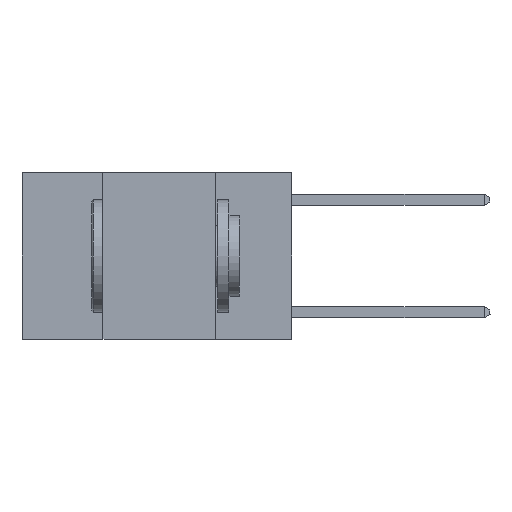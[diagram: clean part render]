
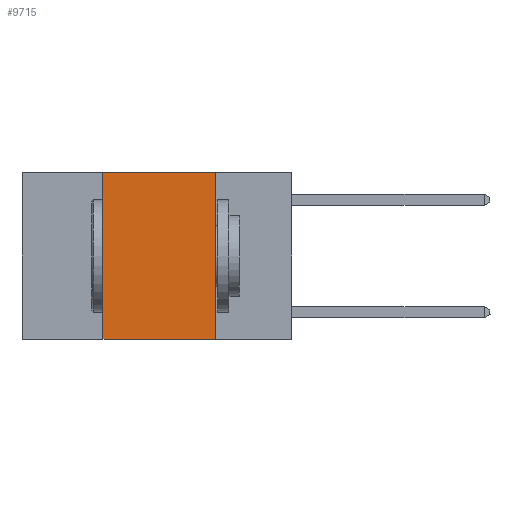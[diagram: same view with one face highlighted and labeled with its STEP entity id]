
A CAD part, left-side view. The second image highlights one B-rep face of the part: STEP entity #9715.
In plain terms, the highlighted planar face has unit normal (-1, 0, 0).
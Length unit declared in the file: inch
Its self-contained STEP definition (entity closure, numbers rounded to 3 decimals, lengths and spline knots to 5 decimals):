
#93 = DIRECTION ( 'NONE',  ( 1., 0., 0. ) ) ;
#131 = LINE ( 'NONE', #6409, #14704 ) ;
#371 = EDGE_LOOP ( 'NONE', ( #15436, #6193, #489, #10617 ) ) ;
#489 = ORIENTED_EDGE ( 'NONE', *, *, #5505, .F. ) ;
#572 = AXIS2_PLACEMENT_3D ( 'NONE', #1726, #93, #17816 ) ;
#579 = LINE ( 'NONE', #14500, #13747 ) ;
#1726 = CARTESIAN_POINT ( 'NONE',  ( 0., 0.6, 0. ) ) ;
#3951 = VERTEX_POINT ( 'NONE', #20063 ) ;
#4758 = CARTESIAN_POINT ( 'NONE',  ( 0., 0.6, -0.37 ) ) ;
#5505 = EDGE_CURVE ( 'NONE', #15310, #16180, #8501, .T. ) ;
#5695 = VERTEX_POINT ( 'NONE', #18073 ) ;
#6193 = ORIENTED_EDGE ( 'NONE', *, *, #14468, .F. ) ;
#6409 = CARTESIAN_POINT ( 'NONE',  ( 0., 0.17, 0. ) ) ;
#6821 = DIRECTION ( 'NONE',  ( 0., 0., 1. ) ) ;
#7764 = DIRECTION ( 'NONE',  ( 0., -1., 0. ) ) ;
#8501 = LINE ( 'NONE', #9853, #15175 ) ;
#8723 = EDGE_CURVE ( 'NONE', #15310, #3951, #9543, .T. ) ;
#9543 = LINE ( 'NONE', #4758, #10365 ) ;
#9715 = ADVANCED_FACE ( 'NONE', ( #17205 ), #15655, .F. ) ;
#9853 = CARTESIAN_POINT ( 'NONE',  ( 0., 0.42, 0. ) ) ;
#10365 = VECTOR ( 'NONE', #7764, 39.37008 ) ;
#10617 = ORIENTED_EDGE ( 'NONE', *, *, #8723, .T. ) ;
#11538 = DIRECTION ( 'NONE',  ( 0., -1., 0. ) ) ;
#12345 = EDGE_CURVE ( 'NONE', #5695, #3951, #131, .T. ) ;
#13747 = VECTOR ( 'NONE', #11538, 39.37008 ) ;
#13803 = CARTESIAN_POINT ( 'NONE',  ( 0., 0.42, -0.37 ) ) ;
#14357 = DIRECTION ( 'NONE',  ( 0., 0., -1. ) ) ;
#14468 = EDGE_CURVE ( 'NONE', #16180, #5695, #579, .T. ) ;
#14500 = CARTESIAN_POINT ( 'NONE',  ( 0., 0.6, 0. ) ) ;
#14704 = VECTOR ( 'NONE', #14357, 39.37008 ) ;
#15175 = VECTOR ( 'NONE', #6821, 39.37008 ) ;
#15310 = VERTEX_POINT ( 'NONE', #13803 ) ;
#15436 = ORIENTED_EDGE ( 'NONE', *, *, #12345, .F. ) ;
#15655 = PLANE ( 'NONE',  #572 ) ;
#16180 = VERTEX_POINT ( 'NONE', #18373 ) ;
#17205 = FACE_OUTER_BOUND ( 'NONE', #371, .T. ) ;
#17816 = DIRECTION ( 'NONE',  ( 0., 0., -1. ) ) ;
#18073 = CARTESIAN_POINT ( 'NONE',  ( 0., 0.17, 0. ) ) ;
#18373 = CARTESIAN_POINT ( 'NONE',  ( 0., 0.42, 0. ) ) ;
#20063 = CARTESIAN_POINT ( 'NONE',  ( 0., 0.17, -0.37 ) ) ;
